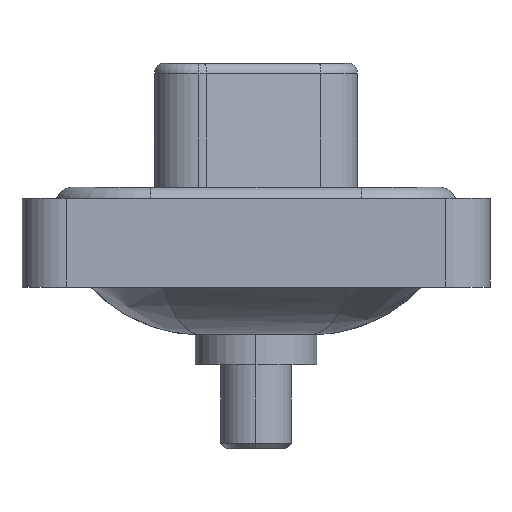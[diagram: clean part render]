
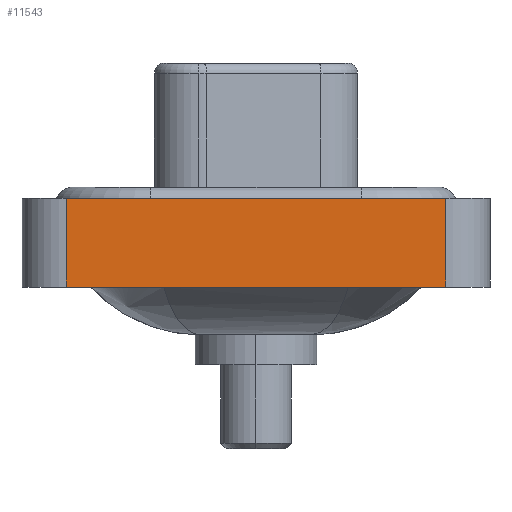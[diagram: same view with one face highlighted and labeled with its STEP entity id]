
A CAD part, left-side view. The second image highlights one B-rep face of the part: STEP entity #11543.
In plain terms, the highlighted planar face has unit normal (-1, 0, 0).
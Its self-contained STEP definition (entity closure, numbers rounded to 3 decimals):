
#304 = CARTESIAN_POINT ( 'NONE',  ( -7.3, 8.55, -3.6 ) ) ;
#430 = EDGE_LOOP ( 'NONE', ( #3114, #656, #4613, #12555 ) ) ;
#606 = DIRECTION ( 'NONE',  ( 0., 0., 1. ) ) ;
#656 = ORIENTED_EDGE ( 'NONE', *, *, #1752, .F. ) ;
#1048 = CARTESIAN_POINT ( 'NONE',  ( -7.3, 8.55, 0.4 ) ) ;
#1752 = EDGE_CURVE ( 'NONE', #12724, #6626, #8003, .T. ) ;
#2652 = VECTOR ( 'NONE', #15495, 1000. ) ;
#3114 = ORIENTED_EDGE ( 'NONE', *, *, #7347, .T. ) ;
#4267 = CARTESIAN_POINT ( 'NONE',  ( -7.3, -8.55, -3.6 ) ) ;
#4357 = DIRECTION ( 'NONE',  ( 0., -1., 0. ) ) ;
#4571 = FACE_OUTER_BOUND ( 'NONE', #430, .T. ) ;
#4613 = ORIENTED_EDGE ( 'NONE', *, *, #6905, .F. ) ;
#4689 = LINE ( 'NONE', #6291, #5027 ) ;
#5027 = VECTOR ( 'NONE', #11354, 1000. ) ;
#5704 = LINE ( 'NONE', #4267, #7945 ) ;
#5979 = CARTESIAN_POINT ( 'NONE',  ( -7.3, -8.55, 0.4 ) ) ;
#6291 = CARTESIAN_POINT ( 'NONE',  ( -7.3, -8.55, -3.6 ) ) ;
#6626 = VERTEX_POINT ( 'NONE', #5979 ) ;
#6905 = EDGE_CURVE ( 'NONE', #11975, #12724, #16247, .T. ) ;
#7165 = EDGE_CURVE ( 'NONE', #11975, #11116, #5704, .T. ) ;
#7347 = EDGE_CURVE ( 'NONE', #11116, #6626, #4689, .T. ) ;
#7886 = AXIS2_PLACEMENT_3D ( 'NONE', #11897, #10743, #606 ) ;
#7945 = VECTOR ( 'NONE', #4357, 1000. ) ;
#8003 = LINE ( 'NONE', #13080, #10590 ) ;
#9513 = CARTESIAN_POINT ( 'NONE',  ( -7.3, -8.55, -3.6 ) ) ;
#10590 = VECTOR ( 'NONE', #15632, 1000. ) ;
#10743 = DIRECTION ( 'NONE',  ( -1., 0., 0. ) ) ;
#11116 = VERTEX_POINT ( 'NONE', #9513 ) ;
#11354 = DIRECTION ( 'NONE',  ( 0., 0., 1. ) ) ;
#11543 = ADVANCED_FACE ( 'NONE', ( #4571 ), #15622, .T. ) ;
#11897 = CARTESIAN_POINT ( 'NONE',  ( -7.3, -8.55, -3.6 ) ) ;
#11975 = VERTEX_POINT ( 'NONE', #15363 ) ;
#12555 = ORIENTED_EDGE ( 'NONE', *, *, #7165, .T. ) ;
#12724 = VERTEX_POINT ( 'NONE', #1048 ) ;
#13080 = CARTESIAN_POINT ( 'NONE',  ( -7.3, -8.55, 0.4 ) ) ;
#15363 = CARTESIAN_POINT ( 'NONE',  ( -7.3, 8.55, -3.6 ) ) ;
#15495 = DIRECTION ( 'NONE',  ( 0., 0., 1. ) ) ;
#15622 = PLANE ( 'NONE',  #7886 ) ;
#15632 = DIRECTION ( 'NONE',  ( 0., -1., 0. ) ) ;
#16247 = LINE ( 'NONE', #304, #2652 ) ;
